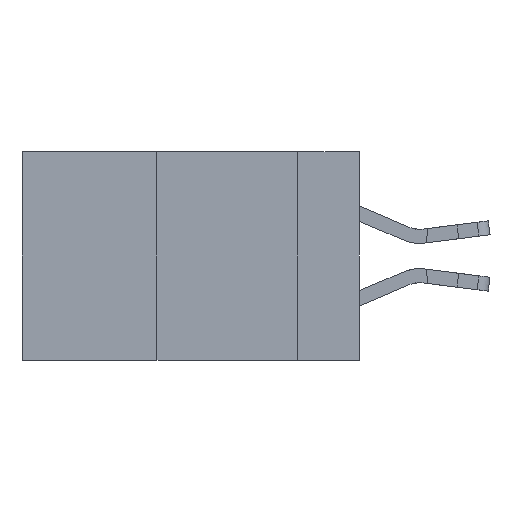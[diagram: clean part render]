
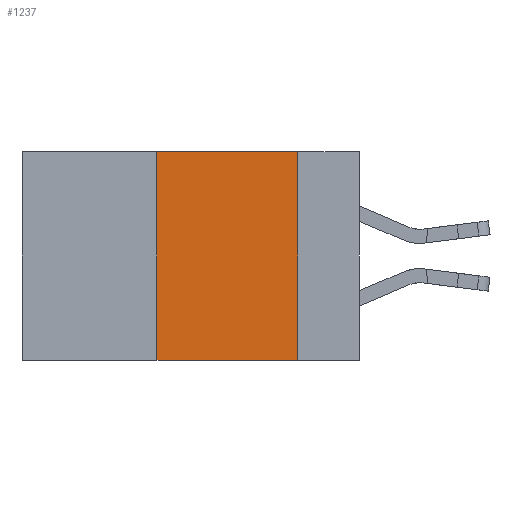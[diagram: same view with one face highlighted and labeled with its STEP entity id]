
A CAD part, left-side view. The second image highlights one B-rep face of the part: STEP entity #1237.
In plain terms, the highlighted planar face has unit normal (-1, 0, 0).
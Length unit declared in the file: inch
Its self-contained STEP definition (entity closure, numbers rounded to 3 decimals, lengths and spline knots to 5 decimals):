
#499 = VECTOR ( 'NONE', #7894, 39.37008 ) ;
#1237 = ADVANCED_FACE ( 'NONE', ( #8339 ), #24154, .F. ) ;
#1636 = VERTEX_POINT ( 'NONE', #2612 ) ;
#2612 = CARTESIAN_POINT ( 'NONE',  ( 0., 0.36, 0. ) ) ;
#4346 = VECTOR ( 'NONE', #9199, 39.37008 ) ;
#5317 = CARTESIAN_POINT ( 'NONE',  ( 0., 0.36, -0.37 ) ) ;
#6399 = DIRECTION ( 'NONE',  ( 0., 0., -1. ) ) ;
#7264 = VERTEX_POINT ( 'NONE', #5317 ) ;
#7718 = CARTESIAN_POINT ( 'NONE',  ( 0., 0.11, 0. ) ) ;
#7894 = DIRECTION ( 'NONE',  ( 0., 0., 1. ) ) ;
#8021 = LINE ( 'NONE', #17536, #499 ) ;
#8163 = VERTEX_POINT ( 'NONE', #7718 ) ;
#8339 = FACE_OUTER_BOUND ( 'NONE', #23277, .T. ) ;
#8399 = EDGE_CURVE ( 'NONE', #7264, #16328, #18722, .T. ) ;
#8634 = EDGE_CURVE ( 'NONE', #1636, #8163, #21916, .T. ) ;
#9199 = DIRECTION ( 'NONE',  ( 0., -1., 0. ) ) ;
#9960 = CARTESIAN_POINT ( 'NONE',  ( 0., 0.6, 0. ) ) ;
#11624 = LINE ( 'NONE', #15618, #15294 ) ;
#12032 = ORIENTED_EDGE ( 'NONE', *, *, #16597, .F. ) ;
#13581 = ORIENTED_EDGE ( 'NONE', *, *, #16587, .F. ) ;
#13828 = DIRECTION ( 'NONE',  ( 0., -1., 0. ) ) ;
#14395 = CARTESIAN_POINT ( 'NONE',  ( 0., 0.6, 0. ) ) ;
#15131 = CARTESIAN_POINT ( 'NONE',  ( 0., 0.6, -0.37 ) ) ;
#15294 = VECTOR ( 'NONE', #25373, 39.37008 ) ;
#15479 = VECTOR ( 'NONE', #13828, 39.37008 ) ;
#15618 = CARTESIAN_POINT ( 'NONE',  ( 0., 0.11, 0. ) ) ;
#16202 = DIRECTION ( 'NONE',  ( 1., 0., 0. ) ) ;
#16328 = VERTEX_POINT ( 'NONE', #24296 ) ;
#16587 = EDGE_CURVE ( 'NONE', #7264, #1636, #8021, .T. ) ;
#16597 = EDGE_CURVE ( 'NONE', #8163, #16328, #11624, .T. ) ;
#17536 = CARTESIAN_POINT ( 'NONE',  ( 0., 0.36, 0. ) ) ;
#18722 = LINE ( 'NONE', #15131, #4346 ) ;
#21277 = ORIENTED_EDGE ( 'NONE', *, *, #8634, .F. ) ;
#21832 = ORIENTED_EDGE ( 'NONE', *, *, #8399, .T. ) ;
#21916 = LINE ( 'NONE', #9960, #15479 ) ;
#22637 = AXIS2_PLACEMENT_3D ( 'NONE', #14395, #16202, #6399 ) ;
#23277 = EDGE_LOOP ( 'NONE', ( #12032, #21277, #13581, #21832 ) ) ;
#24154 = PLANE ( 'NONE',  #22637 ) ;
#24296 = CARTESIAN_POINT ( 'NONE',  ( 0., 0.11, -0.37 ) ) ;
#25373 = DIRECTION ( 'NONE',  ( 0., 0., -1. ) ) ;
